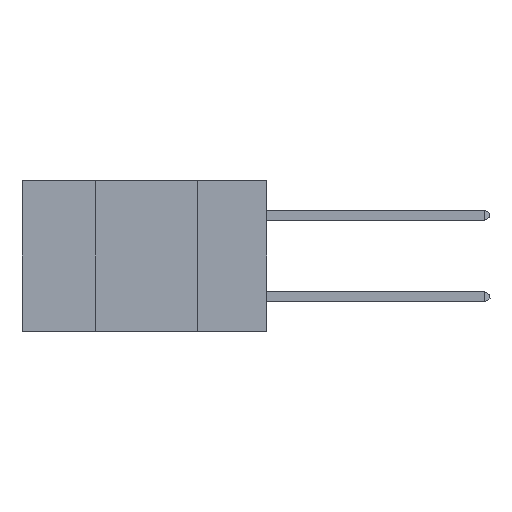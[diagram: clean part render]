
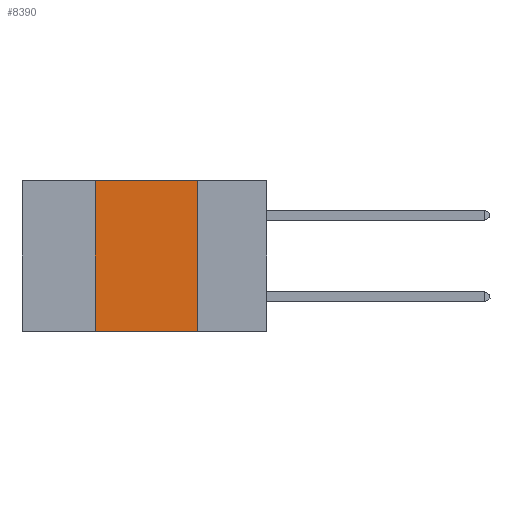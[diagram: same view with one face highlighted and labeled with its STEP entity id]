
A CAD part, left-side view. The second image highlights one B-rep face of the part: STEP entity #8390.
In plain terms, the highlighted planar face has unit normal (-1, 0, 0).
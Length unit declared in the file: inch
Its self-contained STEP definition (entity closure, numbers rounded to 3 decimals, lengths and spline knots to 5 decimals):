
#499 = DIRECTION ( 'NONE',  ( 1., 0., 0. ) ) ;
#763 = DIRECTION ( 'NONE',  ( 0., -1., 0. ) ) ;
#2008 = VERTEX_POINT ( 'NONE', #3483 ) ;
#2150 = VECTOR ( 'NONE', #763, 39.37008 ) ;
#2210 = CARTESIAN_POINT ( 'NONE',  ( 0., 0.17, 0. ) ) ;
#2272 = LINE ( 'NONE', #15850, #13437 ) ;
#2302 = CARTESIAN_POINT ( 'NONE',  ( 0., 0.6, 0. ) ) ;
#2977 = VERTEX_POINT ( 'NONE', #11339 ) ;
#3483 = CARTESIAN_POINT ( 'NONE',  ( 0., 0.42, 0. ) ) ;
#4071 = EDGE_LOOP ( 'NONE', ( #10565, #11520, #7063, #10155 ) ) ;
#4885 = AXIS2_PLACEMENT_3D ( 'NONE', #7616, #499, #10819 ) ;
#5950 = DIRECTION ( 'NONE',  ( 0., 0., 1. ) ) ;
#6144 = LINE ( 'NONE', #2302, #2150 ) ;
#6195 = CARTESIAN_POINT ( 'NONE',  ( 0., 0.6, -0.37 ) ) ;
#7063 = ORIENTED_EDGE ( 'NONE', *, *, #17779, .F. ) ;
#7210 = EDGE_CURVE ( 'NONE', #10809, #14250, #7771, .T. ) ;
#7616 = CARTESIAN_POINT ( 'NONE',  ( 0., 0.6, 0. ) ) ;
#7621 = EDGE_CURVE ( 'NONE', #2977, #14250, #14689, .T. ) ;
#7637 = DIRECTION ( 'NONE',  ( 0., -1., 0. ) ) ;
#7771 = LINE ( 'NONE', #2210, #8214 ) ;
#7973 = CARTESIAN_POINT ( 'NONE',  ( 0., 0.17, 0. ) ) ;
#8214 = VECTOR ( 'NONE', #12430, 39.37008 ) ;
#8378 = FACE_OUTER_BOUND ( 'NONE', #4071, .T. ) ;
#8390 = ADVANCED_FACE ( 'NONE', ( #8378 ), #9363, .F. ) ;
#8518 = EDGE_CURVE ( 'NONE', #2008, #10809, #6144, .T. ) ;
#9363 = PLANE ( 'NONE',  #4885 ) ;
#10057 = CARTESIAN_POINT ( 'NONE',  ( 0., 0.17, -0.37 ) ) ;
#10155 = ORIENTED_EDGE ( 'NONE', *, *, #7621, .T. ) ;
#10565 = ORIENTED_EDGE ( 'NONE', *, *, #7210, .F. ) ;
#10809 = VERTEX_POINT ( 'NONE', #7973 ) ;
#10819 = DIRECTION ( 'NONE',  ( 0., 0., -1. ) ) ;
#11339 = CARTESIAN_POINT ( 'NONE',  ( 0., 0.42, -0.37 ) ) ;
#11520 = ORIENTED_EDGE ( 'NONE', *, *, #8518, .F. ) ;
#12430 = DIRECTION ( 'NONE',  ( 0., 0., -1. ) ) ;
#13437 = VECTOR ( 'NONE', #5950, 39.37008 ) ;
#14250 = VERTEX_POINT ( 'NONE', #10057 ) ;
#14689 = LINE ( 'NONE', #6195, #17986 ) ;
#15850 = CARTESIAN_POINT ( 'NONE',  ( 0., 0.42, 0. ) ) ;
#17779 = EDGE_CURVE ( 'NONE', #2977, #2008, #2272, .T. ) ;
#17986 = VECTOR ( 'NONE', #7637, 39.37008 ) ;
